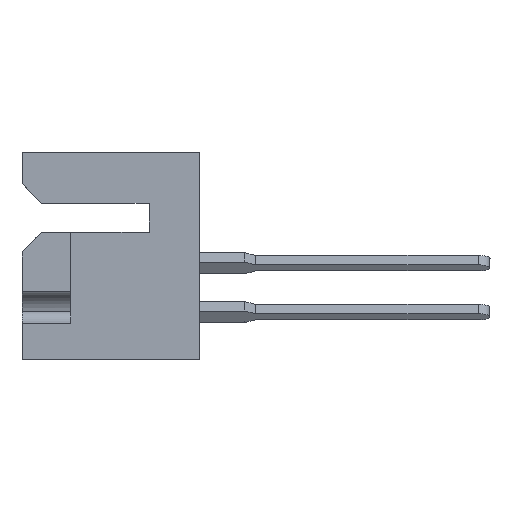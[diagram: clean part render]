
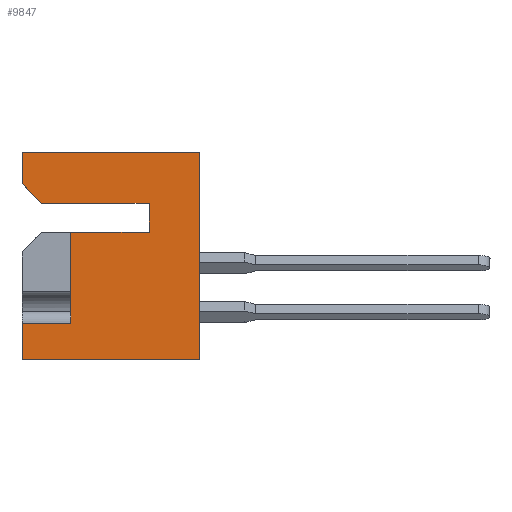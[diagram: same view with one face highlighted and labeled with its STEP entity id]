
A CAD part, left-side view. The second image highlights one B-rep face of the part: STEP entity #9847.
In plain terms, the highlighted planar face has unit normal (-1, 0, 0).
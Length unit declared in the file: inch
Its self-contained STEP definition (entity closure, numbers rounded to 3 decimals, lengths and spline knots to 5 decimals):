
#105 = EDGE_CURVE ( 'NONE', #9161, #8817, #7966, .T. ) ;
#331 = LINE ( 'NONE', #6946, #2737 ) ;
#347 = VECTOR ( 'NONE', #8585, 39.37008 ) ;
#541 = CARTESIAN_POINT ( 'NONE',  ( 0., 0.453, 0. ) ) ;
#594 = CARTESIAN_POINT ( 'NONE',  ( 0., 0.128, -0.205 ) ) ;
#1152 = CARTESIAN_POINT ( 'NONE',  ( 0., 0.453, -0.081 ) ) ;
#1437 = VERTEX_POINT ( 'NONE', #17857 ) ;
#1646 = CARTESIAN_POINT ( 'NONE',  ( 0., 0.403, -0.131 ) ) ;
#1798 = LINE ( 'NONE', #17073, #13673 ) ;
#2099 = EDGE_CURVE ( 'NONE', #1437, #13802, #3947, .T. ) ;
#2647 = ORIENTED_EDGE ( 'NONE', *, *, #8315, .T. ) ;
#2737 = VECTOR ( 'NONE', #8519, 39.37008 ) ;
#3302 = VECTOR ( 'NONE', #3746, 39.37008 ) ;
#3335 = ORIENTED_EDGE ( 'NONE', *, *, #15820, .T. ) ;
#3362 = CARTESIAN_POINT ( 'NONE',  ( 0., 0.328, -0.437 ) ) ;
#3699 = ORIENTED_EDGE ( 'NONE', *, *, #8345, .F. ) ;
#3746 = DIRECTION ( 'NONE',  ( 0., 0., 1. ) ) ;
#3931 = LINE ( 'NONE', #594, #11729 ) ;
#3947 = LINE ( 'NONE', #12182, #14378 ) ;
#4010 = CARTESIAN_POINT ( 'NONE',  ( 0., 0.128, -0.131 ) ) ;
#4250 = FACE_OUTER_BOUND ( 'NONE', #12217, .T. ) ;
#4454 = LINE ( 'NONE', #17684, #347 ) ;
#4659 = PLANE ( 'NONE',  #10183 ) ;
#5188 = VERTEX_POINT ( 'NONE', #8648 ) ;
#5221 = ORIENTED_EDGE ( 'NONE', *, *, #6086, .F. ) ;
#5311 = EDGE_CURVE ( 'NONE', #15682, #9161, #9931, .T. ) ;
#5672 = LINE ( 'NONE', #4010, #12216 ) ;
#5764 = CARTESIAN_POINT ( 'NONE',  ( 0., 0.453, 0. ) ) ;
#6086 = EDGE_CURVE ( 'NONE', #9121, #6414, #10643, .T. ) ;
#6138 = DIRECTION ( 'NONE',  ( 0., 0., 1. ) ) ;
#6215 = CARTESIAN_POINT ( 'NONE',  ( 0., 0.453, 0. ) ) ;
#6414 = VERTEX_POINT ( 'NONE', #19603 ) ;
#6851 = EDGE_CURVE ( 'NONE', #15373, #12330, #15405, .T. ) ;
#6946 = CARTESIAN_POINT ( 'NONE',  ( 0., 0.328, -0.437 ) ) ;
#7247 = CARTESIAN_POINT ( 'NONE',  ( 0., 0.403, -0.131 ) ) ;
#7966 = LINE ( 'NONE', #541, #9169 ) ;
#8315 = EDGE_CURVE ( 'NONE', #9121, #5188, #4454, .T. ) ;
#8345 = EDGE_CURVE ( 'NONE', #12593, #1437, #5672, .T. ) ;
#8405 = EDGE_CURVE ( 'NONE', #15373, #6414, #331, .T. ) ;
#8519 = DIRECTION ( 'NONE',  ( 0., 1., 0. ) ) ;
#8585 = DIRECTION ( 'NONE',  ( 0., -1., 0. ) ) ;
#8599 = EDGE_CURVE ( 'NONE', #15682, #13802, #17252, .T. ) ;
#8648 = CARTESIAN_POINT ( 'NONE',  ( 0., 0., -0.531 ) ) ;
#8817 = VERTEX_POINT ( 'NONE', #11212 ) ;
#9121 = VERTEX_POINT ( 'NONE', #10651 ) ;
#9159 = DIRECTION ( 'NONE',  ( 0., 0., 1. ) ) ;
#9161 = VERTEX_POINT ( 'NONE', #5764 ) ;
#9169 = VECTOR ( 'NONE', #16160, 39.37008 ) ;
#9847 = ADVANCED_FACE ( 'NONE', ( #4250 ), #4659, .F. ) ;
#9931 = LINE ( 'NONE', #14984, #15257 ) ;
#9998 = DIRECTION ( 'NONE',  ( 0., 0., 1. ) ) ;
#10183 = AXIS2_PLACEMENT_3D ( 'NONE', #6215, #15475, #17017 ) ;
#10643 = LINE ( 'NONE', #11834, #18344 ) ;
#10651 = CARTESIAN_POINT ( 'NONE',  ( 0., 0.453, -0.531 ) ) ;
#10662 = ORIENTED_EDGE ( 'NONE', *, *, #2099, .F. ) ;
#10901 = DIRECTION ( 'NONE',  ( 0., 1., 0. ) ) ;
#11212 = CARTESIAN_POINT ( 'NONE',  ( 0., 0., 0. ) ) ;
#11729 = VECTOR ( 'NONE', #17279, 39.37008 ) ;
#11834 = CARTESIAN_POINT ( 'NONE',  ( 0., 0.453, 0. ) ) ;
#12182 = CARTESIAN_POINT ( 'NONE',  ( 0., 0.128, -0.131 ) ) ;
#12216 = VECTOR ( 'NONE', #9998, 39.37008 ) ;
#12217 = EDGE_LOOP ( 'NONE', ( #14049, #5221, #2647, #3335, #18571, #13299, #14501, #10662, #3699, #14904, #15261 ) ) ;
#12330 = VERTEX_POINT ( 'NONE', #13524 ) ;
#12496 = DIRECTION ( 'NONE',  ( 0., -0.707, -0.707 ) ) ;
#12593 = VERTEX_POINT ( 'NONE', #18904 ) ;
#13169 = VECTOR ( 'NONE', #12496, 39.37008 ) ;
#13299 = ORIENTED_EDGE ( 'NONE', *, *, #5311, .F. ) ;
#13524 = CARTESIAN_POINT ( 'NONE',  ( 0., 0.328, -0.205 ) ) ;
#13673 = VECTOR ( 'NONE', #6138, 39.37008 ) ;
#13802 = VERTEX_POINT ( 'NONE', #7247 ) ;
#14049 = ORIENTED_EDGE ( 'NONE', *, *, #8405, .T. ) ;
#14378 = VECTOR ( 'NONE', #10901, 39.37008 ) ;
#14501 = ORIENTED_EDGE ( 'NONE', *, *, #8599, .T. ) ;
#14904 = ORIENTED_EDGE ( 'NONE', *, *, #17285, .T. ) ;
#14984 = CARTESIAN_POINT ( 'NONE',  ( 0., 0.453, 0. ) ) ;
#15257 = VECTOR ( 'NONE', #18143, 39.37008 ) ;
#15261 = ORIENTED_EDGE ( 'NONE', *, *, #6851, .F. ) ;
#15373 = VERTEX_POINT ( 'NONE', #3362 ) ;
#15405 = LINE ( 'NONE', #17484, #3302 ) ;
#15475 = DIRECTION ( 'NONE',  ( 1., 0., 0. ) ) ;
#15682 = VERTEX_POINT ( 'NONE', #1152 ) ;
#15820 = EDGE_CURVE ( 'NONE', #5188, #8817, #1798, .T. ) ;
#16160 = DIRECTION ( 'NONE',  ( 0., -1., 0. ) ) ;
#17017 = DIRECTION ( 'NONE',  ( 0., 0., -1. ) ) ;
#17073 = CARTESIAN_POINT ( 'NONE',  ( 0., 0., 0. ) ) ;
#17252 = LINE ( 'NONE', #1646, #13169 ) ;
#17279 = DIRECTION ( 'NONE',  ( 0., 1., 0. ) ) ;
#17285 = EDGE_CURVE ( 'NONE', #12593, #12330, #3931, .T. ) ;
#17484 = CARTESIAN_POINT ( 'NONE',  ( 0., 0.328, -0.205 ) ) ;
#17684 = CARTESIAN_POINT ( 'NONE',  ( 0., 0.453, -0.531 ) ) ;
#17857 = CARTESIAN_POINT ( 'NONE',  ( 0., 0.128, -0.131 ) ) ;
#18143 = DIRECTION ( 'NONE',  ( 0., 0., 1. ) ) ;
#18344 = VECTOR ( 'NONE', #9159, 39.37008 ) ;
#18571 = ORIENTED_EDGE ( 'NONE', *, *, #105, .F. ) ;
#18904 = CARTESIAN_POINT ( 'NONE',  ( 0., 0.128, -0.205 ) ) ;
#19603 = CARTESIAN_POINT ( 'NONE',  ( 0., 0.453, -0.437 ) ) ;
